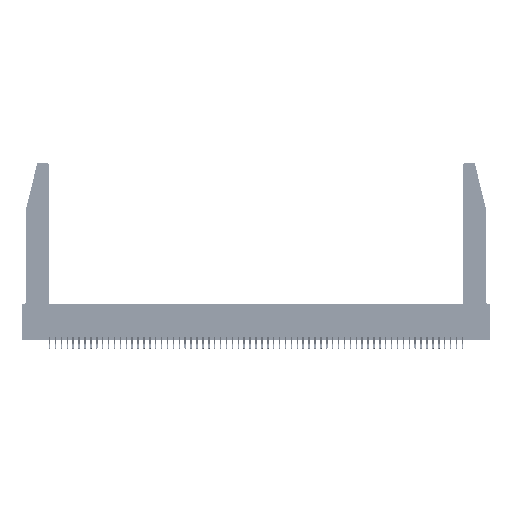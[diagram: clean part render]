
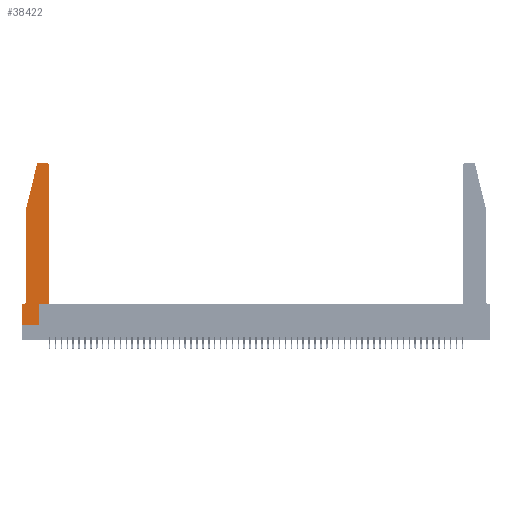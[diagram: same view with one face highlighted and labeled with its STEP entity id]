
A CAD part, top view. The second image highlights one B-rep face of the part: STEP entity #38422.
In plain terms, the highlighted planar face has unit normal (0, 0, 1).
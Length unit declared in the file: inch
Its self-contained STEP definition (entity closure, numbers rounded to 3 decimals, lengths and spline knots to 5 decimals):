
#1240 = VERTEX_POINT ( 'NONE', #52959 ) ;
#1288 = EDGE_CURVE ( 'NONE', #39999, #3274, #7009, .T. ) ;
#2654 = AXIS2_PLACEMENT_3D ( 'NONE', #54078, #32201, #23400 ) ;
#3274 = VERTEX_POINT ( 'NONE', #22595 ) ;
#4904 = DIRECTION ( 'NONE',  ( 0., 0., 1. ) ) ;
#5282 = EDGE_CURVE ( 'NONE', #49376, #46890, #53829, .T. ) ;
#5554 = VERTEX_POINT ( 'NONE', #10066 ) ;
#6201 = LINE ( 'NONE', #12732, #16502 ) ;
#6564 = EDGE_CURVE ( 'NONE', #46890, #18743, #28378, .T. ) ;
#6778 = VERTEX_POINT ( 'NONE', #14148 ) ;
#7009 = CIRCLE ( 'NONE', #2654, 0.03 ) ;
#7662 = LINE ( 'NONE', #29391, #14552 ) ;
#8233 = DIRECTION ( 'NONE',  ( -0.239, -0.971, 0. ) ) ;
#8650 = ORIENTED_EDGE ( 'NONE', *, *, #33640, .T. ) ;
#9143 = CARTESIAN_POINT ( 'NONE',  ( 0.4505, 0.35, 0.37 ) ) ;
#10066 = CARTESIAN_POINT ( 'NONE',  ( 0., 0.35, 0.37 ) ) ;
#11622 = CIRCLE ( 'NONE', #32820, 0.07 ) ;
#12732 = CARTESIAN_POINT ( 'NONE',  ( 0., 0., 0.37 ) ) ;
#12762 = CARTESIAN_POINT ( 'NONE',  ( 0.4505, 0.35, 0.37 ) ) ;
#13142 = CARTESIAN_POINT ( 'NONE',  ( 0.2865, 0.35, 0.37 ) ) ;
#13625 = DIRECTION ( 'NONE',  ( 0., 1., 0. ) ) ;
#13974 = VECTOR ( 'NONE', #8233, 39.37008 ) ;
#14148 = CARTESIAN_POINT ( 'NONE',  ( 0.2865, 0., 0.37 ) ) ;
#14552 = VECTOR ( 'NONE', #15632, 39.37008 ) ;
#15169 = DIRECTION ( 'NONE',  ( 0., 0., -1. ) ) ;
#15280 = AXIS2_PLACEMENT_3D ( 'NONE', #31124, #4904, #35557 ) ;
#15470 = CARTESIAN_POINT ( 'NONE',  ( 0.0755, 0.42, 0.37 ) ) ;
#15632 = DIRECTION ( 'NONE',  ( -1., 0., 0. ) ) ;
#16267 = VECTOR ( 'NONE', #22387, 39.37008 ) ;
#16502 = VECTOR ( 'NONE', #34962, 39.37008 ) ;
#16529 = ORIENTED_EDGE ( 'NONE', *, *, #39579, .T. ) ;
#17197 = DIRECTION ( 'NONE',  ( 1., 0., 0. ) ) ;
#18743 = VERTEX_POINT ( 'NONE', #49282 ) ;
#19405 = VECTOR ( 'NONE', #13625, 39.37008 ) ;
#19570 = DIRECTION ( 'NONE',  ( -1., 0., 0. ) ) ;
#20997 = VECTOR ( 'NONE', #41461, 39.37008 ) ;
#21224 = LINE ( 'NONE', #37373, #37046 ) ;
#21419 = LINE ( 'NONE', #53151, #19405 ) ;
#22387 = DIRECTION ( 'NONE',  ( 0., 1., 0. ) ) ;
#22595 = CARTESIAN_POINT ( 'NONE',  ( 0.4205, 2.75, 0.37 ) ) ;
#23186 = CARTESIAN_POINT ( 'NONE',  ( 0.2605, 2.75, 0.37 ) ) ;
#23400 = DIRECTION ( 'NONE',  ( 1., 0., 0. ) ) ;
#24299 = VERTEX_POINT ( 'NONE', #13142 ) ;
#24343 = VECTOR ( 'NONE', #26949, 39.37008 ) ;
#24714 = VERTEX_POINT ( 'NONE', #38016 ) ;
#26732 = ORIENTED_EDGE ( 'NONE', *, *, #45893, .T. ) ;
#26949 = DIRECTION ( 'NONE',  ( 1., 0., 0. ) ) ;
#27792 = VECTOR ( 'NONE', #53879, 39.37008 ) ;
#28378 = LINE ( 'NONE', #34492, #13974 ) ;
#28699 = DIRECTION ( 'NONE',  ( 1., 0., 0. ) ) ;
#29213 = CARTESIAN_POINT ( 'NONE',  ( 0.4505, 2.72, 0.37 ) ) ;
#29391 = CARTESIAN_POINT ( 'NONE',  ( 0.0755, 0.35, 0.37 ) ) ;
#29823 = ORIENTED_EDGE ( 'NONE', *, *, #6564, .T. ) ;
#30933 = PLANE ( 'NONE',  #15280 ) ;
#31124 = CARTESIAN_POINT ( 'NONE',  ( 0., 0.35, 0.37 ) ) ;
#31538 = ORIENTED_EDGE ( 'NONE', *, *, #34145, .T. ) ;
#32201 = DIRECTION ( 'NONE',  ( 0., 0., 1. ) ) ;
#32633 = CARTESIAN_POINT ( 'NONE',  ( 0.0055, 0.42, 0.37 ) ) ;
#32636 = CARTESIAN_POINT ( 'NONE',  ( 0.0755, 2., 0.37 ) ) ;
#32712 = LINE ( 'NONE', #32636, #20997 ) ;
#32820 = AXIS2_PLACEMENT_3D ( 'NONE', #32633, #15169, #19570 ) ;
#32860 = VERTEX_POINT ( 'NONE', #54194 ) ;
#33640 = EDGE_CURVE ( 'NONE', #18743, #44170, #32712, .T. ) ;
#34145 = EDGE_CURVE ( 'NONE', #3274, #49376, #44283, .T. ) ;
#34492 = CARTESIAN_POINT ( 'NONE',  ( 0.0755, 2., 0.37 ) ) ;
#34568 = EDGE_CURVE ( 'NONE', #24299, #24714, #47672, .T. ) ;
#34962 = DIRECTION ( 'NONE',  ( 0., -1., 0. ) ) ;
#35557 = DIRECTION ( 'NONE',  ( 1., 0., 0. ) ) ;
#37046 = VECTOR ( 'NONE', #28699, 39.37008 ) ;
#37226 = EDGE_CURVE ( 'NONE', #44170, #32860, #11622, .T. ) ;
#37373 = CARTESIAN_POINT ( 'NONE',  ( 0., 0., 0.37 ) ) ;
#37780 = ORIENTED_EDGE ( 'NONE', *, *, #1288, .T. ) ;
#38016 = CARTESIAN_POINT ( 'NONE',  ( 0.4505, 0.35, 0.37 ) ) ;
#38422 = ADVANCED_FACE ( 'NONE', ( #40420 ), #30933, .T. ) ;
#39579 = EDGE_CURVE ( 'NONE', #24714, #39999, #51935, .T. ) ;
#39999 = VERTEX_POINT ( 'NONE', #29213 ) ;
#40420 = FACE_OUTER_BOUND ( 'NONE', #52614, .T. ) ;
#41003 = ORIENTED_EDGE ( 'NONE', *, *, #55722, .T. ) ;
#41341 = CARTESIAN_POINT ( 'NONE',  ( 0.284, 2.75, 0.37 ) ) ;
#41345 = EDGE_CURVE ( 'NONE', #1240, #6778, #21224, .T. ) ;
#41461 = DIRECTION ( 'NONE',  ( 0., -1., 0. ) ) ;
#44170 = VERTEX_POINT ( 'NONE', #15470 ) ;
#44283 = LINE ( 'NONE', #23186, #27792 ) ;
#45893 = EDGE_CURVE ( 'NONE', #32860, #5554, #7662, .T. ) ;
#46890 = VERTEX_POINT ( 'NONE', #52957 ) ;
#47672 = LINE ( 'NONE', #12762, #24343 ) ;
#48282 = CARTESIAN_POINT ( 'NONE',  ( 0.284, 2.72, 0.37 ) ) ;
#48687 = AXIS2_PLACEMENT_3D ( 'NONE', #48282, #52503, #17197 ) ;
#49282 = CARTESIAN_POINT ( 'NONE',  ( 0.0755, 2., 0.37 ) ) ;
#49376 = VERTEX_POINT ( 'NONE', #41341 ) ;
#50480 = ORIENTED_EDGE ( 'NONE', *, *, #34568, .T. ) ;
#51089 = ORIENTED_EDGE ( 'NONE', *, *, #37226, .T. ) ;
#51098 = ORIENTED_EDGE ( 'NONE', *, *, #5282, .T. ) ;
#51935 = LINE ( 'NONE', #9143, #16267 ) ;
#52503 = DIRECTION ( 'NONE',  ( 0., 0., 1. ) ) ;
#52614 = EDGE_LOOP ( 'NONE', ( #31538, #51098, #29823, #8650, #51089, #26732, #41003, #52930, #54982, #50480, #16529, #37780 ) ) ;
#52930 = ORIENTED_EDGE ( 'NONE', *, *, #41345, .T. ) ;
#52957 = CARTESIAN_POINT ( 'NONE',  ( 0.25487, 2.72718, 0.37 ) ) ;
#52959 = CARTESIAN_POINT ( 'NONE',  ( 0., 0., 0.37 ) ) ;
#53151 = CARTESIAN_POINT ( 'NONE',  ( 0.2865, 0.35, 0.37 ) ) ;
#53829 = CIRCLE ( 'NONE', #48687, 0.03 ) ;
#53879 = DIRECTION ( 'NONE',  ( -1., 0., 0. ) ) ;
#54078 = CARTESIAN_POINT ( 'NONE',  ( 0.4205, 2.72, 0.37 ) ) ;
#54194 = CARTESIAN_POINT ( 'NONE',  ( 0.0055, 0.35, 0.37 ) ) ;
#54550 = EDGE_CURVE ( 'NONE', #6778, #24299, #21419, .T. ) ;
#54982 = ORIENTED_EDGE ( 'NONE', *, *, #54550, .T. ) ;
#55722 = EDGE_CURVE ( 'NONE', #5554, #1240, #6201, .T. ) ;
